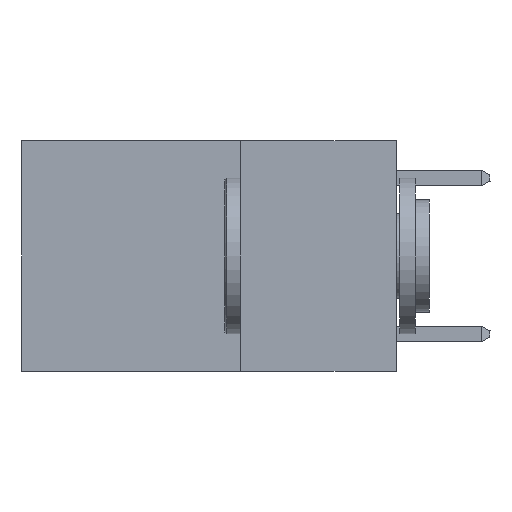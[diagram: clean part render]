
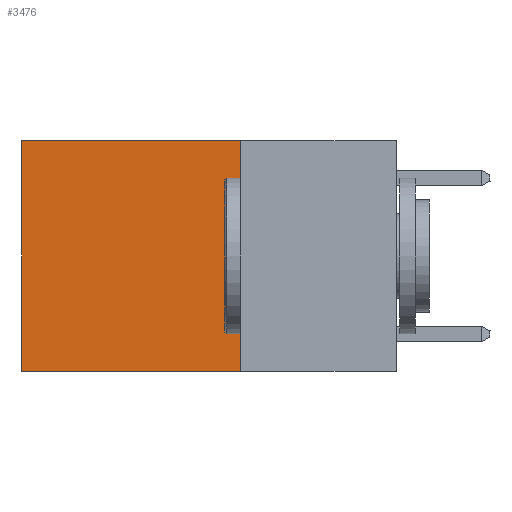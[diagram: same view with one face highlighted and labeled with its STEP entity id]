
A CAD part, left-side view. The second image highlights one B-rep face of the part: STEP entity #3476.
In plain terms, the highlighted planar face has unit normal (-1, 0, 0).
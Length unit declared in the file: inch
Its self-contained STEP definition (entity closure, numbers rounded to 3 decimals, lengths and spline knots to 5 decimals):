
#98 = VECTOR ( 'NONE', #1875, 39.37008 ) ;
#165 = VECTOR ( 'NONE', #2398, 39.37008 ) ;
#434 = ORIENTED_EDGE ( 'NONE', *, *, #7567, .F. ) ;
#475 = LINE ( 'NONE', #4260, #9944 ) ;
#766 = AXIS2_PLACEMENT_3D ( 'NONE', #4281, #1135, #5153 ) ;
#824 = CARTESIAN_POINT ( 'NONE',  ( 0.2625, 0.25, 0. ) ) ;
#1135 = DIRECTION ( 'NONE',  ( 1., 0., 0. ) ) ;
#1875 = DIRECTION ( 'NONE',  ( 0., 0., -1. ) ) ;
#2398 = DIRECTION ( 'NONE',  ( 0., 0., -1. ) ) ;
#2803 = LINE ( 'NONE', #10075, #4016 ) ;
#2845 = EDGE_LOOP ( 'NONE', ( #3829, #434, #7353, #4950 ) ) ;
#3082 = LINE ( 'NONE', #8121, #165 ) ;
#3281 = FACE_OUTER_BOUND ( 'NONE', #2845, .T. ) ;
#3476 = ADVANCED_FACE ( 'NONE', ( #3281 ), #5369, .F. ) ;
#3815 = DIRECTION ( 'NONE',  ( 0., 1., 0. ) ) ;
#3829 = ORIENTED_EDGE ( 'NONE', *, *, #8186, .T. ) ;
#4016 = VECTOR ( 'NONE', #3815, 39.37008 ) ;
#4260 = CARTESIAN_POINT ( 'NONE',  ( 0.2625, 0.25, 0. ) ) ;
#4281 = CARTESIAN_POINT ( 'NONE',  ( 0.2625, 0.25, 0. ) ) ;
#4518 = EDGE_CURVE ( 'NONE', #6442, #5874, #475, .T. ) ;
#4918 = EDGE_CURVE ( 'NONE', #6442, #9565, #3082, .T. ) ;
#4950 = ORIENTED_EDGE ( 'NONE', *, *, #4518, .T. ) ;
#5045 = CARTESIAN_POINT ( 'NONE',  ( 0.2625, 0.25, -0.37 ) ) ;
#5153 = DIRECTION ( 'NONE',  ( 0., 0., -1. ) ) ;
#5357 = CARTESIAN_POINT ( 'NONE',  ( 0.2625, 0.6, -0.37 ) ) ;
#5369 = PLANE ( 'NONE',  #766 ) ;
#5874 = VERTEX_POINT ( 'NONE', #8652 ) ;
#6153 = LINE ( 'NONE', #9837, #98 ) ;
#6442 = VERTEX_POINT ( 'NONE', #824 ) ;
#6645 = DIRECTION ( 'NONE',  ( 0., 1., 0. ) ) ;
#7353 = ORIENTED_EDGE ( 'NONE', *, *, #4918, .F. ) ;
#7444 = VERTEX_POINT ( 'NONE', #5357 ) ;
#7567 = EDGE_CURVE ( 'NONE', #9565, #7444, #2803, .T. ) ;
#8121 = CARTESIAN_POINT ( 'NONE',  ( 0.2625, 0.25, 0. ) ) ;
#8186 = EDGE_CURVE ( 'NONE', #5874, #7444, #6153, .T. ) ;
#8652 = CARTESIAN_POINT ( 'NONE',  ( 0.2625, 0.6, 0. ) ) ;
#9565 = VERTEX_POINT ( 'NONE', #5045 ) ;
#9837 = CARTESIAN_POINT ( 'NONE',  ( 0.2625, 0.6, 0. ) ) ;
#9944 = VECTOR ( 'NONE', #6645, 39.37008 ) ;
#10075 = CARTESIAN_POINT ( 'NONE',  ( 0.2625, 0.25, -0.37 ) ) ;
